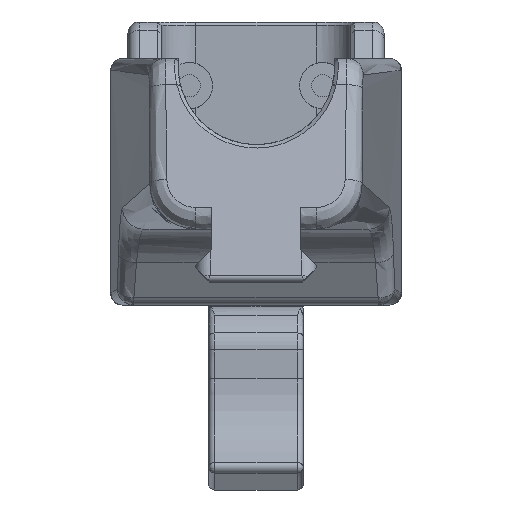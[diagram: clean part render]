
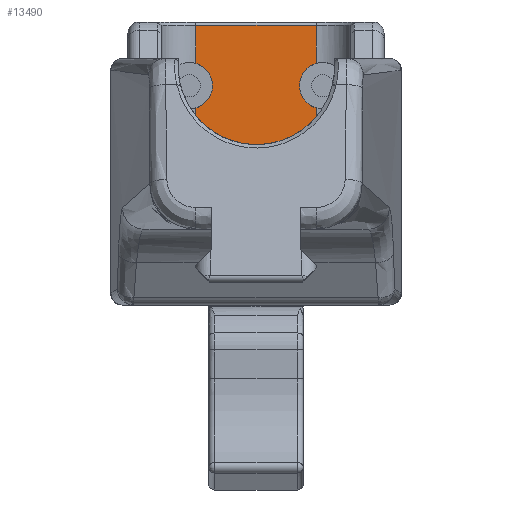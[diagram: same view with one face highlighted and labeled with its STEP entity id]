
A CAD part, front view. The second image highlights one B-rep face of the part: STEP entity #13490.
In plain terms, the highlighted planar face has unit normal (0, -1, 0).
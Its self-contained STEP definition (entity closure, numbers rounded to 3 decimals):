
#975=CIRCLE('',#14682,4.);
#976=CIRCLE('',#14683,4.);
#977=CIRCLE('',#14684,4.);
#1337=PLANE('',#14681);
#2062=FACE_OUTER_BOUND('',#2868,.T.);
#2868=EDGE_LOOP('',(#12070,#12071,#12072,#12073,#12074,#12075,#12076,#12077,
#12078));
#3911=LINE('',#27783,#4997);
#3960=LINE('',#28012,#5046);
#3961=LINE('',#28041,#5047);
#3962=LINE('',#28047,#5048);
#3963=LINE('',#28078,#5049);
#3964=LINE('',#28080,#5050);
#4997=VECTOR('',#17806,10.);
#5046=VECTOR('',#17961,10.);
#5047=VECTOR('',#17962,10.);
#5048=VECTOR('',#17969,10.);
#5049=VECTOR('',#17970,10.);
#5050=VECTOR('',#17973,10.);
#6391=VERTEX_POINT('',#27772);
#6394=VERTEX_POINT('',#27781);
#6442=VERTEX_POINT('',#28011);
#6443=VERTEX_POINT('',#28013);
#6444=VERTEX_POINT('',#28040);
#6445=VERTEX_POINT('',#28044);
#6446=VERTEX_POINT('',#28046);
#6448=VERTEX_POINT('',#28063);
#6449=VERTEX_POINT('',#28083);
#8274=EDGE_CURVE('',#6394,#6391,#3911,.T.);
#8354=EDGE_CURVE('',#6391,#6442,#3960,.T.);
#8356=EDGE_CURVE('',#6443,#6444,#3961,.T.);
#8359=EDGE_CURVE('',#6445,#6446,#3962,.T.);
#8362=EDGE_CURVE('',#6448,#6394,#3963,.T.);
#8363=EDGE_CURVE('',#6445,#6444,#3964,.F.);
#8364=EDGE_CURVE('',#6448,#6446,#975,.F.);
#8365=EDGE_CURVE('',#6443,#6449,#976,.F.);
#8366=EDGE_CURVE('',#6449,#6442,#977,.F.);
#12070=ORIENTED_EDGE('',*,*,#8274,.F.);
#12071=ORIENTED_EDGE('',*,*,#8362,.F.);
#12072=ORIENTED_EDGE('',*,*,#8364,.T.);
#12073=ORIENTED_EDGE('',*,*,#8359,.F.);
#12074=ORIENTED_EDGE('',*,*,#8363,.T.);
#12075=ORIENTED_EDGE('',*,*,#8356,.F.);
#12076=ORIENTED_EDGE('',*,*,#8365,.T.);
#12077=ORIENTED_EDGE('',*,*,#8366,.T.);
#12078=ORIENTED_EDGE('',*,*,#8354,.F.);
#13490=ADVANCED_FACE('',(#2062),#1337,.T.);
#14681=AXIS2_PLACEMENT_3D('',#28081,#17974,#17975);
#14682=AXIS2_PLACEMENT_3D('',#28082,#17976,#17977);
#14683=AXIS2_PLACEMENT_3D('',#28084,#17978,#17979);
#14684=AXIS2_PLACEMENT_3D('',#28085,#17980,#17981);
#17806=DIRECTION('',(1.,0.,0.));
#17961=DIRECTION('',(0.,0.,-1.));
#17962=DIRECTION('',(0.,0.,-1.));
#17969=DIRECTION('',(0.,0.,1.));
#17970=DIRECTION('',(0.,0.,1.));
#17973=DIRECTION('',(-1.,0.,0.));
#17974=DIRECTION('center_axis',(0.,-1.,0.));
#17975=DIRECTION('ref_axis',(1.,0.,0.));
#17976=DIRECTION('center_axis',(0.,-1.,0.));
#17977=DIRECTION('ref_axis',(1.,0.,0.));
#17978=DIRECTION('center_axis',(0.,-1.,0.));
#17979=DIRECTION('ref_axis',(1.,0.,0.));
#17980=DIRECTION('center_axis',(0.,-1.,0.));
#17981=DIRECTION('ref_axis',(1.,0.,0.));
#27772=CARTESIAN_POINT('',(26.353,138.082,-109.189));
#27781=CARTESIAN_POINT('',(5.6,138.082,-109.189));
#27783=CARTESIAN_POINT('',(7.788,138.082,-109.189));
#28011=CARTESIAN_POINT('',(26.353,138.082,-115.727));
#28012=CARTESIAN_POINT('',(26.353,138.082,-136.589));
#28013=CARTESIAN_POINT('',(26.353,138.082,-123.411));
#28040=CARTESIAN_POINT('',(26.353,138.082,-136.889));
#28041=CARTESIAN_POINT('',(26.353,138.082,-136.589));
#28044=CARTESIAN_POINT('',(5.6,138.082,-136.889));
#28046=CARTESIAN_POINT('',(5.6,138.082,-123.411));
#28047=CARTESIAN_POINT('',(5.6,138.082,-136.589));
#28063=CARTESIAN_POINT('',(5.6,138.082,-115.727));
#28078=CARTESIAN_POINT('',(5.6,138.082,-136.589));
#28080=CARTESIAN_POINT('',(7.788,138.082,-136.889));
#28081=CARTESIAN_POINT('Origin',(-0.4,138.082,-136.589));
#28082=CARTESIAN_POINT('Origin',(4.487,138.082,-119.569));
#28083=CARTESIAN_POINT('',(23.466,138.082,-119.569));
#28084=CARTESIAN_POINT('Origin',(27.466,138.082,-119.569));
#28085=CARTESIAN_POINT('Origin',(27.466,138.082,-119.569));
